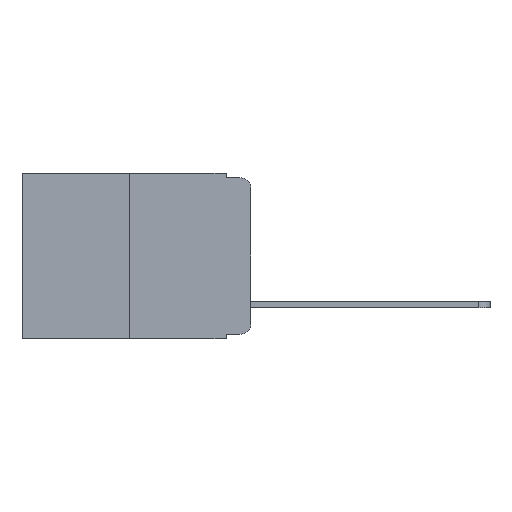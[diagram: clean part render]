
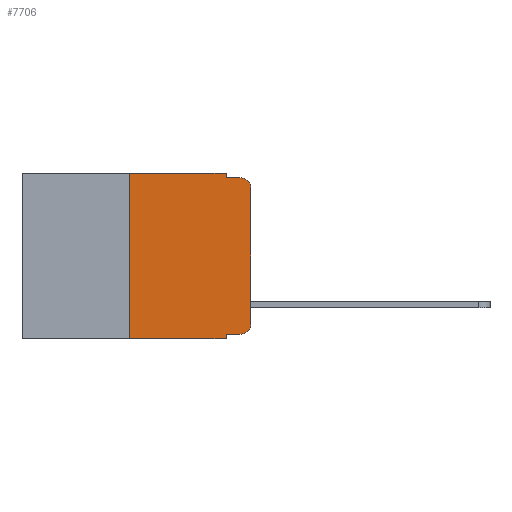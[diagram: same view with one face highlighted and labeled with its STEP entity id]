
A CAD part, left-side view. The second image highlights one B-rep face of the part: STEP entity #7706.
In plain terms, the highlighted planar face has unit normal (-1, 0, 0).
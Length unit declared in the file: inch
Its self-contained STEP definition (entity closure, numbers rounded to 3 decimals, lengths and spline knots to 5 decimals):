
#35 = CARTESIAN_POINT ( 'NONE',  ( 0., 0.473, 0. ) ) ;
#54 = EDGE_LOOP ( 'NONE', ( #2796, #3010, #3242, #4099, #4465, #4604, #4912, #5308, #6147, #7521 ) ) ;
#710 = DIRECTION ( 'NONE',  ( 0., -1., 0. ) ) ;
#1098 = VERTEX_POINT ( 'NONE', #5812 ) ;
#1315 = DIRECTION ( 'NONE',  ( 0., 0., -1. ) ) ;
#1659 = VECTOR ( 'NONE', #1315, 39.37008 ) ;
#1737 = DIRECTION ( 'NONE',  ( 0., 0., -1. ) ) ;
#1859 = DIRECTION ( 'NONE',  ( -1., 0., 0. ) ) ;
#1886 = EDGE_CURVE ( 'NONE', #5563, #4469, #9540, .T. ) ;
#2057 = VECTOR ( 'NONE', #2616, 39.37008 ) ;
#2060 = DIRECTION ( 'NONE',  ( 0., 0., 1. ) ) ;
#2205 = FACE_OUTER_BOUND ( 'NONE', #54, .T. ) ;
#2431 = EDGE_CURVE ( 'NONE', #5179, #10341, #2625, .T. ) ;
#2459 = CARTESIAN_POINT ( 'NONE',  ( 0., 0., -0.03 ) ) ;
#2560 = LINE ( 'NONE', #3728, #11924 ) ;
#2576 = EDGE_CURVE ( 'NONE', #7556, #2758, #3859, .T. ) ;
#2612 = CARTESIAN_POINT ( 'NONE',  ( 0., 0.051, 0. ) ) ;
#2616 = DIRECTION ( 'NONE',  ( 0., 0., -1. ) ) ;
#2625 = LINE ( 'NONE', #4257, #5045 ) ;
#2729 = VERTEX_POINT ( 'NONE', #6579 ) ;
#2758 = VERTEX_POINT ( 'NONE', #6446 ) ;
#2796 = ORIENTED_EDGE ( 'NONE', *, *, #2431, .T. ) ;
#2919 = DIRECTION ( 'NONE',  ( 0., 0., 1. ) ) ;
#3010 = ORIENTED_EDGE ( 'NONE', *, *, #3310, .T. ) ;
#3192 = DIRECTION ( 'NONE',  ( 0., 0., -1. ) ) ;
#3242 = ORIENTED_EDGE ( 'NONE', *, *, #3637, .F. ) ;
#3256 = CARTESIAN_POINT ( 'NONE',  ( 0., 0.473, -0.343 ) ) ;
#3285 = AXIS2_PLACEMENT_3D ( 'NONE', #8901, #8753, #8915 ) ;
#3310 = EDGE_CURVE ( 'NONE', #10341, #2729, #6054, .T. ) ;
#3504 = DIRECTION ( 'NONE',  ( 0., -1., 0. ) ) ;
#3637 = EDGE_CURVE ( 'NONE', #1098, #2729, #5311, .T. ) ;
#3728 = CARTESIAN_POINT ( 'NONE',  ( 0., 0.051, -0.333 ) ) ;
#3835 = EDGE_CURVE ( 'NONE', #2758, #1098, #9364, .T. ) ;
#3859 = LINE ( 'NONE', #35, #6378 ) ;
#4099 = ORIENTED_EDGE ( 'NONE', *, *, #3835, .F. ) ;
#4134 = PLANE ( 'NONE',  #10838 ) ;
#4159 = VERTEX_POINT ( 'NONE', #8077 ) ;
#4257 = CARTESIAN_POINT ( 'NONE',  ( 0., 0., 0. ) ) ;
#4344 = EDGE_CURVE ( 'NONE', #5563, #7556, #10435, .T. ) ;
#4465 = ORIENTED_EDGE ( 'NONE', *, *, #2576, .F. ) ;
#4469 = VERTEX_POINT ( 'NONE', #7913 ) ;
#4470 = CARTESIAN_POINT ( 'NONE',  ( 0., 0.02, -0.03 ) ) ;
#4480 = EDGE_CURVE ( 'NONE', #4159, #4469, #11332, .T. ) ;
#4604 = ORIENTED_EDGE ( 'NONE', *, *, #4344, .F. ) ;
#4628 = EDGE_CURVE ( 'NONE', #4159, #10323, #2560, .T. ) ;
#4665 = EDGE_CURVE ( 'NONE', #10323, #5179, #5289, .T. ) ;
#4912 = ORIENTED_EDGE ( 'NONE', *, *, #1886, .T. ) ;
#5045 = VECTOR ( 'NONE', #2919, 39.37008 ) ;
#5179 = VERTEX_POINT ( 'NONE', #11673 ) ;
#5289 = CIRCLE ( 'NONE', #3285, 0.02 ) ;
#5308 = ORIENTED_EDGE ( 'NONE', *, *, #4480, .F. ) ;
#5311 = LINE ( 'NONE', #8296, #10314 ) ;
#5563 = VERTEX_POINT ( 'NONE', #11430 ) ;
#5812 = CARTESIAN_POINT ( 'NONE',  ( 0., 0.051, -0.01 ) ) ;
#6054 = CIRCLE ( 'NONE', #6618, 0.02 ) ;
#6147 = ORIENTED_EDGE ( 'NONE', *, *, #4628, .T. ) ;
#6316 = CARTESIAN_POINT ( 'NONE',  ( 0., 0.25, 0. ) ) ;
#6378 = VECTOR ( 'NONE', #710, 39.37008 ) ;
#6446 = CARTESIAN_POINT ( 'NONE',  ( 0., 0.051, 0. ) ) ;
#6579 = CARTESIAN_POINT ( 'NONE',  ( 0., 0.02, -0.01 ) ) ;
#6618 = AXIS2_PLACEMENT_3D ( 'NONE', #4470, #1859, #1737 ) ;
#6863 = DIRECTION ( 'NONE',  ( 0., -1., 0. ) ) ;
#7146 = DIRECTION ( 'NONE',  ( 0., -1., 0. ) ) ;
#7521 = ORIENTED_EDGE ( 'NONE', *, *, #4665, .T. ) ;
#7556 = VERTEX_POINT ( 'NONE', #6316 ) ;
#7706 = ADVANCED_FACE ( 'NONE', ( #2205 ), #4134, .F. ) ;
#7913 = CARTESIAN_POINT ( 'NONE',  ( 0., 0.051, -0.343 ) ) ;
#8077 = CARTESIAN_POINT ( 'NONE',  ( 0., 0.051, -0.333 ) ) ;
#8296 = CARTESIAN_POINT ( 'NONE',  ( 0., 0.051, -0.01 ) ) ;
#8753 = DIRECTION ( 'NONE',  ( -1., 0., 0. ) ) ;
#8901 = CARTESIAN_POINT ( 'NONE',  ( 0., 0.02, -0.313 ) ) ;
#8915 = DIRECTION ( 'NONE',  ( 0., 0., -1. ) ) ;
#9129 = CARTESIAN_POINT ( 'NONE',  ( 0., 0.473, 0. ) ) ;
#9244 = DIRECTION ( 'NONE',  ( 1., 0., 0. ) ) ;
#9260 = VECTOR ( 'NONE', #6863, 39.37008 ) ;
#9364 = LINE ( 'NONE', #2612, #2057 ) ;
#9540 = LINE ( 'NONE', #3256, #9260 ) ;
#9847 = CARTESIAN_POINT ( 'NONE',  ( 0., 0.051, 0. ) ) ;
#9898 = CARTESIAN_POINT ( 'NONE',  ( 0., 0.02, -0.333 ) ) ;
#10314 = VECTOR ( 'NONE', #7146, 39.37008 ) ;
#10323 = VERTEX_POINT ( 'NONE', #9898 ) ;
#10341 = VERTEX_POINT ( 'NONE', #2459 ) ;
#10435 = LINE ( 'NONE', #11643, #12058 ) ;
#10838 = AXIS2_PLACEMENT_3D ( 'NONE', #9129, #9244, #3192 ) ;
#11332 = LINE ( 'NONE', #9847, #1659 ) ;
#11430 = CARTESIAN_POINT ( 'NONE',  ( 0., 0.25, -0.343 ) ) ;
#11643 = CARTESIAN_POINT ( 'NONE',  ( 0., 0.25, 0. ) ) ;
#11673 = CARTESIAN_POINT ( 'NONE',  ( 0., 0., -0.313 ) ) ;
#11924 = VECTOR ( 'NONE', #3504, 39.37008 ) ;
#12058 = VECTOR ( 'NONE', #2060, 39.37008 ) ;
